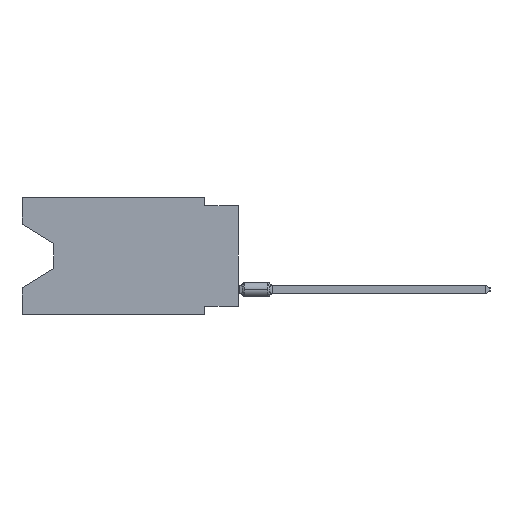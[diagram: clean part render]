
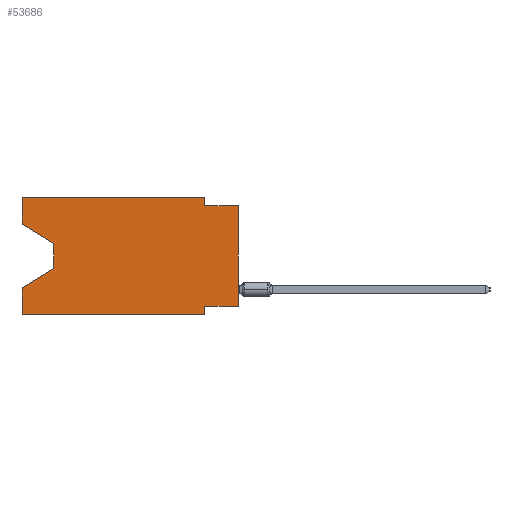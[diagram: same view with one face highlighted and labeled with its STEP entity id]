
A CAD part, left-side view. The second image highlights one B-rep face of the part: STEP entity #53686.
In plain terms, the highlighted planar face has unit normal (-1, 0, 0).
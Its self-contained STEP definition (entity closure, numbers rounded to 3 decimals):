
#334 = LINE ( 'NONE', #32561, #70277 ) ;
#690 = CARTESIAN_POINT ( 'NONE',  ( 0., 0., -8.255 ) ) ;
#1662 = CARTESIAN_POINT ( 'NONE',  ( 0., 2.54, 0. ) ) ;
#3134 = VERTEX_POINT ( 'NONE', #92037 ) ;
#4807 = CARTESIAN_POINT ( 'NONE',  ( 0., 2.54, -8.255 ) ) ;
#5489 = LINE ( 'NONE', #88898, #6350 ) ;
#6350 = VECTOR ( 'NONE', #57640, 1000. ) ;
#8324 = DIRECTION ( 'NONE',  ( 0., -0.855, -0.519 ) ) ;
#10295 = DIRECTION ( 'NONE',  ( 0., -1., 0. ) ) ;
#10385 = DIRECTION ( 'NONE',  ( 0., 0., 1. ) ) ;
#10536 = VECTOR ( 'NONE', #8324, 1000. ) ;
#13772 = EDGE_CURVE ( 'NONE', #73969, #19708, #40005, .T. ) ;
#14050 = CARTESIAN_POINT ( 'NONE',  ( 0., 16.383, -2.038 ) ) ;
#14867 = EDGE_CURVE ( 'NONE', #83372, #47883, #5489, .T. ) ;
#14874 = CARTESIAN_POINT ( 'NONE',  ( 0., 16.383, -8.89 ) ) ;
#15164 = ORIENTED_EDGE ( 'NONE', *, *, #14867, .T. ) ;
#16017 = CARTESIAN_POINT ( 'NONE',  ( 0., 2.54, -0.635 ) ) ;
#16733 = DIRECTION ( 'NONE',  ( 0., -1., 0. ) ) ;
#16839 = EDGE_CURVE ( 'NONE', #85710, #78929, #96400, .T. ) ;
#17579 = EDGE_CURVE ( 'NONE', #19708, #76291, #49040, .T. ) ;
#17668 = VERTEX_POINT ( 'NONE', #71865 ) ;
#19417 = VECTOR ( 'NONE', #10295, 1000. ) ;
#19708 = VERTEX_POINT ( 'NONE', #78123 ) ;
#20117 = ORIENTED_EDGE ( 'NONE', *, *, #57949, .F. ) ;
#20360 = LINE ( 'NONE', #50170, #78904 ) ;
#21722 = ORIENTED_EDGE ( 'NONE', *, *, #17579, .F. ) ;
#21760 = LINE ( 'NONE', #46072, #10536 ) ;
#22362 = LINE ( 'NONE', #29828, #82597 ) ;
#23193 = CARTESIAN_POINT ( 'NONE',  ( 0., 16.383, -8.89 ) ) ;
#24417 = CARTESIAN_POINT ( 'NONE',  ( 0., 16.383, 0. ) ) ;
#27482 = EDGE_CURVE ( 'NONE', #75384, #3134, #69024, .T. ) ;
#28402 = CARTESIAN_POINT ( 'NONE',  ( 0., 2.54, -8.89 ) ) ;
#28482 = EDGE_CURVE ( 'NONE', #73969, #83372, #21760, .T. ) ;
#29828 = CARTESIAN_POINT ( 'NONE',  ( 0., 2.54, 0. ) ) ;
#32561 = CARTESIAN_POINT ( 'NONE',  ( 0., 0., -8.255 ) ) ;
#33415 = EDGE_CURVE ( 'NONE', #75384, #85710, #334, .T. ) ;
#34254 = CARTESIAN_POINT ( 'NONE',  ( 0., 13.97, -3.505 ) ) ;
#37109 = AXIS2_PLACEMENT_3D ( 'NONE', #24417, #94759, #57067 ) ;
#38709 = DIRECTION ( 'NONE',  ( 0., 0., -1. ) ) ;
#39843 = LINE ( 'NONE', #46805, #69644 ) ;
#40005 = LINE ( 'NONE', #46010, #61907 ) ;
#40743 = VECTOR ( 'NONE', #10385, 1000. ) ;
#44103 = ORIENTED_EDGE ( 'NONE', *, *, #16839, .F. ) ;
#46010 = CARTESIAN_POINT ( 'NONE',  ( 0., 16.383, 0. ) ) ;
#46072 = CARTESIAN_POINT ( 'NONE',  ( 0., 16.383, -2.038 ) ) ;
#46110 = ORIENTED_EDGE ( 'NONE', *, *, #87523, .T. ) ;
#46475 = DIRECTION ( 'NONE',  ( 0., 1., 0. ) ) ;
#46805 = CARTESIAN_POINT ( 'NONE',  ( 0., 0., -0.635 ) ) ;
#47883 = VERTEX_POINT ( 'NONE', #82798 ) ;
#49040 = LINE ( 'NONE', #94669, #19417 ) ;
#50100 = PLANE ( 'NONE',  #37109 ) ;
#50170 = CARTESIAN_POINT ( 'NONE',  ( 0., 16.383, 0. ) ) ;
#51100 = ORIENTED_EDGE ( 'NONE', *, *, #92907, .F. ) ;
#52773 = EDGE_CURVE ( 'NONE', #62589, #78929, #91208, .T. ) ;
#53686 = ADVANCED_FACE ( 'NONE', ( #95265 ), #50100, .F. ) ;
#57067 = DIRECTION ( 'NONE',  ( 0., 0., -1. ) ) ;
#57640 = DIRECTION ( 'NONE',  ( 0., 0., -1. ) ) ;
#57949 = EDGE_CURVE ( 'NONE', #76291, #79213, #22362, .T. ) ;
#59797 = ORIENTED_EDGE ( 'NONE', *, *, #28482, .T. ) ;
#60138 = ORIENTED_EDGE ( 'NONE', *, *, #76186, .F. ) ;
#61907 = VECTOR ( 'NONE', #70318, 1000. ) ;
#62589 = VERTEX_POINT ( 'NONE', #14874 ) ;
#66842 = CARTESIAN_POINT ( 'NONE',  ( 0., 13.97, -5.385 ) ) ;
#67115 = DIRECTION ( 'NONE',  ( 0., 0., -1. ) ) ;
#69024 = LINE ( 'NONE', #92817, #40743 ) ;
#69644 = VECTOR ( 'NONE', #70633, 1000. ) ;
#70277 = VECTOR ( 'NONE', #46475, 1000. ) ;
#70318 = DIRECTION ( 'NONE',  ( 0., 0., 1. ) ) ;
#70633 = DIRECTION ( 'NONE',  ( 0., -1., 0. ) ) ;
#71865 = CARTESIAN_POINT ( 'NONE',  ( 0., 16.383, -6.852 ) ) ;
#73969 = VERTEX_POINT ( 'NONE', #14050 ) ;
#75157 = ORIENTED_EDGE ( 'NONE', *, *, #27482, .T. ) ;
#75384 = VERTEX_POINT ( 'NONE', #690 ) ;
#76186 = EDGE_CURVE ( 'NONE', #79213, #3134, #39843, .T. ) ;
#76291 = VERTEX_POINT ( 'NONE', #1662 ) ;
#77277 = ORIENTED_EDGE ( 'NONE', *, *, #33415, .F. ) ;
#78123 = CARTESIAN_POINT ( 'NONE',  ( 0., 16.383, 0. ) ) ;
#78153 = VECTOR ( 'NONE', #16733, 1000. ) ;
#78904 = VECTOR ( 'NONE', #78975, 1000. ) ;
#78929 = VERTEX_POINT ( 'NONE', #92587 ) ;
#78975 = DIRECTION ( 'NONE',  ( 0., 0., 1. ) ) ;
#79213 = VERTEX_POINT ( 'NONE', #16017 ) ;
#79520 = VECTOR ( 'NONE', #67115, 1000. ) ;
#79917 = ORIENTED_EDGE ( 'NONE', *, *, #13772, .F. ) ;
#82597 = VECTOR ( 'NONE', #38709, 1000. ) ;
#82704 = LINE ( 'NONE', #66842, #85386 ) ;
#82798 = CARTESIAN_POINT ( 'NONE',  ( 0., 13.97, -5.385 ) ) ;
#83372 = VERTEX_POINT ( 'NONE', #34254 ) ;
#85386 = VECTOR ( 'NONE', #97103, 1000. ) ;
#85710 = VERTEX_POINT ( 'NONE', #4807 ) ;
#87523 = EDGE_CURVE ( 'NONE', #47883, #17668, #82704, .T. ) ;
#88898 = CARTESIAN_POINT ( 'NONE',  ( 0., 13.97, -3.505 ) ) ;
#91208 = LINE ( 'NONE', #23193, #78153 ) ;
#92037 = CARTESIAN_POINT ( 'NONE',  ( 0., 0., -0.635 ) ) ;
#92587 = CARTESIAN_POINT ( 'NONE',  ( 0., 2.54, -8.89 ) ) ;
#92817 = CARTESIAN_POINT ( 'NONE',  ( 0., 0., 0. ) ) ;
#92907 = EDGE_CURVE ( 'NONE', #62589, #17668, #20360, .T. ) ;
#93589 = ORIENTED_EDGE ( 'NONE', *, *, #52773, .T. ) ;
#94669 = CARTESIAN_POINT ( 'NONE',  ( 0., 16.383, 0. ) ) ;
#94759 = DIRECTION ( 'NONE',  ( 1., 0., 0. ) ) ;
#95265 = FACE_OUTER_BOUND ( 'NONE', #95447, .T. ) ;
#95447 = EDGE_LOOP ( 'NONE', ( #59797, #15164, #46110, #51100, #93589, #44103, #77277, #75157, #60138, #20117, #21722, #79917 ) ) ;
#96400 = LINE ( 'NONE', #28402, #79520 ) ;
#97103 = DIRECTION ( 'NONE',  ( 0., 0.855, -0.519 ) ) ;
